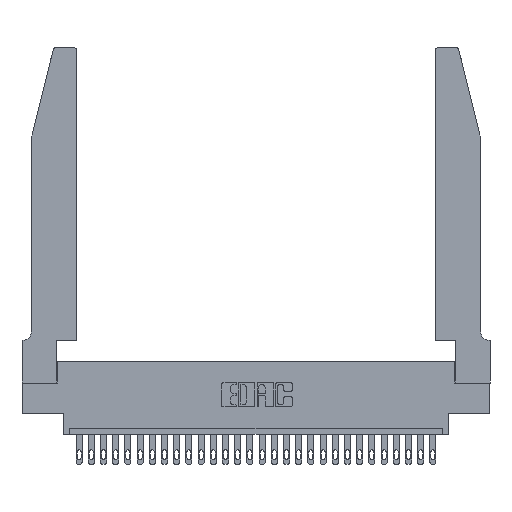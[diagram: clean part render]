
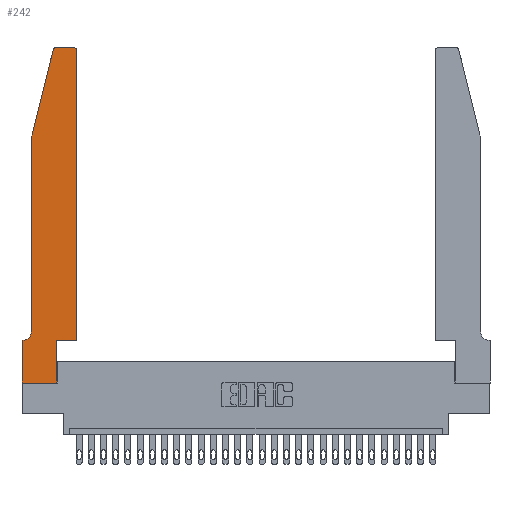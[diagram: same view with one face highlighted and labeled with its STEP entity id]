
A CAD part, top view. The second image highlights one B-rep face of the part: STEP entity #242.
In plain terms, the highlighted planar face has unit normal (0, 0, 1).
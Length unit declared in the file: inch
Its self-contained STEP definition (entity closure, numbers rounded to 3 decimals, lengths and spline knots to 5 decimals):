
#242 = ADVANCED_FACE ( 'NONE', ( #2490 ), #16735, .T. ) ;
#716 = CARTESIAN_POINT ( 'NONE',  ( 0., 0., 0.37 ) ) ;
#892 = ORIENTED_EDGE ( 'NONE', *, *, #23273, .T. ) ;
#907 = CIRCLE ( 'NONE', #4969, 0.07 ) ;
#911 = DIRECTION ( 'NONE',  ( 0., 0., 1. ) ) ;
#1013 = VERTEX_POINT ( 'NONE', #18738 ) ;
#1201 = CARTESIAN_POINT ( 'NONE',  ( 0.2605, 2.75, 0.37 ) ) ;
#1380 = EDGE_CURVE ( 'NONE', #23697, #27478, #28367, .T. ) ;
#1427 = EDGE_CURVE ( 'NONE', #24620, #23313, #7642, .T. ) ;
#1840 = CIRCLE ( 'NONE', #15924, 0.03 ) ;
#2091 = VECTOR ( 'NONE', #9697, 39.37008 ) ;
#2478 = VERTEX_POINT ( 'NONE', #21255 ) ;
#2490 = FACE_OUTER_BOUND ( 'NONE', #6162, .T. ) ;
#2899 = CARTESIAN_POINT ( 'NONE',  ( 0.4505, 2.72, 0.37 ) ) ;
#3054 = CARTESIAN_POINT ( 'NONE',  ( 0.0755, 0.35, 0.37 ) ) ;
#3485 = CARTESIAN_POINT ( 'NONE',  ( 0.2865, 0., 0.37 ) ) ;
#3501 = DIRECTION ( 'NONE',  ( 0., 0., 1. ) ) ;
#4969 = AXIS2_PLACEMENT_3D ( 'NONE', #19437, #10527, #26196 ) ;
#5803 = CARTESIAN_POINT ( 'NONE',  ( 0.2865, 0.35, 0.37 ) ) ;
#5899 = VERTEX_POINT ( 'NONE', #3485 ) ;
#5921 = DIRECTION ( 'NONE',  ( 1., 0., 0. ) ) ;
#6162 = EDGE_LOOP ( 'NONE', ( #19302, #18063, #17550, #7896, #12697, #7190, #12537, #892, #22491, #7067, #25166, #6693 ) ) ;
#6391 = CARTESIAN_POINT ( 'NONE',  ( 0.2865, 0.35, 0.37 ) ) ;
#6693 = ORIENTED_EDGE ( 'NONE', *, *, #1427, .T. ) ;
#7067 = ORIENTED_EDGE ( 'NONE', *, *, #8748, .T. ) ;
#7190 = ORIENTED_EDGE ( 'NONE', *, *, #28896, .T. ) ;
#7455 = DIRECTION ( 'NONE',  ( 0., -1., 0. ) ) ;
#7642 = CIRCLE ( 'NONE', #13708, 0.03 ) ;
#7775 = EDGE_CURVE ( 'NONE', #27478, #26887, #907, .T. ) ;
#7832 = DIRECTION ( 'NONE',  ( -1., 0., 0. ) ) ;
#7896 = ORIENTED_EDGE ( 'NONE', *, *, #1380, .T. ) ;
#8748 = EDGE_CURVE ( 'NONE', #15612, #2478, #16930, .T. ) ;
#8968 = VECTOR ( 'NONE', #21064, 39.37008 ) ;
#9171 = VECTOR ( 'NONE', #27516, 39.37008 ) ;
#9288 = VECTOR ( 'NONE', #16328, 39.37008 ) ;
#9697 = DIRECTION ( 'NONE',  ( -0.239, -0.971, 0. ) ) ;
#10011 = AXIS2_PLACEMENT_3D ( 'NONE', #19107, #911, #25450 ) ;
#10527 = DIRECTION ( 'NONE',  ( 0., 0., -1. ) ) ;
#10610 = DIRECTION ( 'NONE',  ( 0., 1., 0. ) ) ;
#10732 = EDGE_CURVE ( 'NONE', #23313, #23993, #18174, .T. ) ;
#11538 = CARTESIAN_POINT ( 'NONE',  ( 0.0755, 2., 0.37 ) ) ;
#11693 = LINE ( 'NONE', #716, #9288 ) ;
#12253 = CARTESIAN_POINT ( 'NONE',  ( 0.0755, 2., 0.37 ) ) ;
#12343 = VECTOR ( 'NONE', #14955, 39.37008 ) ;
#12537 = ORIENTED_EDGE ( 'NONE', *, *, #23485, .T. ) ;
#12587 = EDGE_CURVE ( 'NONE', #5899, #15612, #13140, .T. ) ;
#12692 = CARTESIAN_POINT ( 'NONE',  ( 0.0755, 0.42, 0.37 ) ) ;
#12697 = ORIENTED_EDGE ( 'NONE', *, *, #7775, .T. ) ;
#13091 = DIRECTION ( 'NONE',  ( 0., 1., 0. ) ) ;
#13140 = LINE ( 'NONE', #5803, #27180 ) ;
#13497 = CARTESIAN_POINT ( 'NONE',  ( 0.4205, 2.75, 0.37 ) ) ;
#13708 = AXIS2_PLACEMENT_3D ( 'NONE', #19247, #3501, #5921 ) ;
#14952 = CARTESIAN_POINT ( 'NONE',  ( 0.4505, 0.35, 0.37 ) ) ;
#14955 = DIRECTION ( 'NONE',  ( 1., 0., 0. ) ) ;
#15612 = VERTEX_POINT ( 'NONE', #6391 ) ;
#15924 = AXIS2_PLACEMENT_3D ( 'NONE', #27009, #22429, #22805 ) ;
#16328 = DIRECTION ( 'NONE',  ( 0., -1., 0. ) ) ;
#16735 = PLANE ( 'NONE',  #10011 ) ;
#16930 = LINE ( 'NONE', #28448, #12343 ) ;
#17445 = CARTESIAN_POINT ( 'NONE',  ( 0.0055, 0.35, 0.37 ) ) ;
#17550 = ORIENTED_EDGE ( 'NONE', *, *, #21002, .T. ) ;
#18063 = ORIENTED_EDGE ( 'NONE', *, *, #20147, .T. ) ;
#18174 = LINE ( 'NONE', #1201, #28412 ) ;
#18581 = CARTESIAN_POINT ( 'NONE',  ( 0.284, 2.75, 0.37 ) ) ;
#18738 = CARTESIAN_POINT ( 'NONE',  ( 0.25487, 2.72718, 0.37 ) ) ;
#19107 = CARTESIAN_POINT ( 'NONE',  ( 0., 0.35, 0.37 ) ) ;
#19195 = EDGE_CURVE ( 'NONE', #2478, #24620, #22055, .T. ) ;
#19247 = CARTESIAN_POINT ( 'NONE',  ( 0.4205, 2.72, 0.37 ) ) ;
#19302 = ORIENTED_EDGE ( 'NONE', *, *, #10732, .T. ) ;
#19437 = CARTESIAN_POINT ( 'NONE',  ( 0.0055, 0.42, 0.37 ) ) ;
#20147 = EDGE_CURVE ( 'NONE', #23993, #1013, #1840, .T. ) ;
#20851 = CARTESIAN_POINT ( 'NONE',  ( 0.0755, 2., 0.37 ) ) ;
#21002 = EDGE_CURVE ( 'NONE', #1013, #23697, #23442, .T. ) ;
#21064 = DIRECTION ( 'NONE',  ( 1., 0., 0. ) ) ;
#21255 = CARTESIAN_POINT ( 'NONE',  ( 0.4505, 0.35, 0.37 ) ) ;
#22055 = LINE ( 'NONE', #14952, #22707 ) ;
#22429 = DIRECTION ( 'NONE',  ( 0., 0., 1. ) ) ;
#22491 = ORIENTED_EDGE ( 'NONE', *, *, #12587, .T. ) ;
#22707 = VECTOR ( 'NONE', #13091, 39.37008 ) ;
#22805 = DIRECTION ( 'NONE',  ( 1., 0., 0. ) ) ;
#23273 = EDGE_CURVE ( 'NONE', #26512, #5899, #24714, .T. ) ;
#23313 = VERTEX_POINT ( 'NONE', #13497 ) ;
#23442 = LINE ( 'NONE', #11538, #2091 ) ;
#23485 = EDGE_CURVE ( 'NONE', #24677, #26512, #11693, .T. ) ;
#23697 = VERTEX_POINT ( 'NONE', #12253 ) ;
#23993 = VERTEX_POINT ( 'NONE', #18581 ) ;
#24620 = VERTEX_POINT ( 'NONE', #2899 ) ;
#24677 = VERTEX_POINT ( 'NONE', #28941 ) ;
#24714 = LINE ( 'NONE', #27726, #8968 ) ;
#24814 = CARTESIAN_POINT ( 'NONE',  ( 0., 0., 0.37 ) ) ;
#25166 = ORIENTED_EDGE ( 'NONE', *, *, #19195, .T. ) ;
#25450 = DIRECTION ( 'NONE',  ( 1., 0., 0. ) ) ;
#26196 = DIRECTION ( 'NONE',  ( -1., 0., 0. ) ) ;
#26512 = VERTEX_POINT ( 'NONE', #24814 ) ;
#26887 = VERTEX_POINT ( 'NONE', #17445 ) ;
#27009 = CARTESIAN_POINT ( 'NONE',  ( 0.284, 2.72, 0.37 ) ) ;
#27180 = VECTOR ( 'NONE', #10610, 39.37008 ) ;
#27478 = VERTEX_POINT ( 'NONE', #12692 ) ;
#27516 = DIRECTION ( 'NONE',  ( -1., 0., 0. ) ) ;
#27621 = VECTOR ( 'NONE', #7455, 39.37008 ) ;
#27726 = CARTESIAN_POINT ( 'NONE',  ( 0., 0., 0.37 ) ) ;
#28367 = LINE ( 'NONE', #20851, #27621 ) ;
#28412 = VECTOR ( 'NONE', #7832, 39.37008 ) ;
#28448 = CARTESIAN_POINT ( 'NONE',  ( 0.4505, 0.35, 0.37 ) ) ;
#28485 = LINE ( 'NONE', #3054, #9171 ) ;
#28896 = EDGE_CURVE ( 'NONE', #26887, #24677, #28485, .T. ) ;
#28941 = CARTESIAN_POINT ( 'NONE',  ( 0., 0.35, 0.37 ) ) ;
